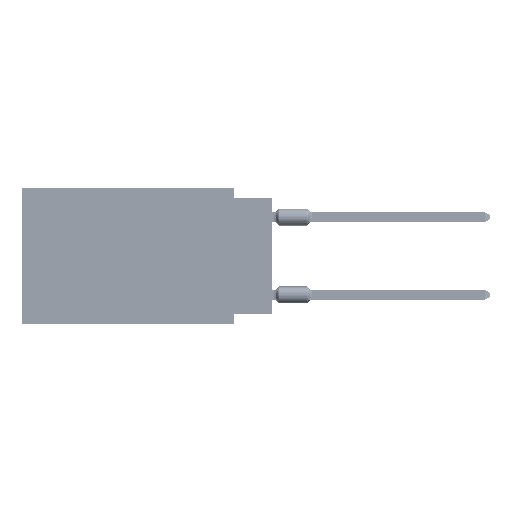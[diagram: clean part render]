
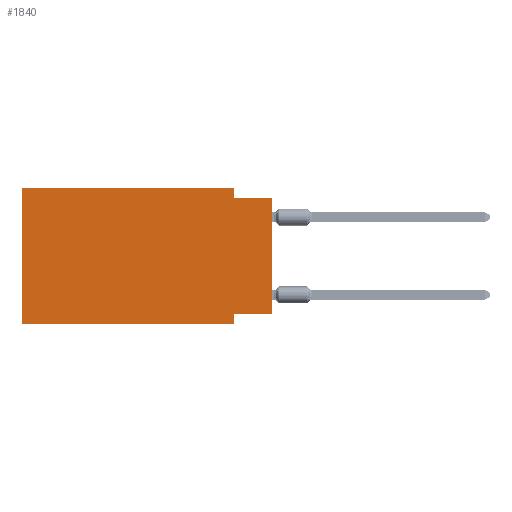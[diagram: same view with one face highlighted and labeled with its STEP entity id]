
A CAD part, left-side view. The second image highlights one B-rep face of the part: STEP entity #1840.
In plain terms, the highlighted planar face has unit normal (-1, 0, 0).
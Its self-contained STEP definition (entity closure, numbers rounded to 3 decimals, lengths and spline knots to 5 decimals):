
#1728 = DIRECTION ( 'NONE',  ( 0., 0., -1. ) ) ;
#1840 = ADVANCED_FACE ( 'NONE', ( #55163 ), #37522, .F. ) ;
#11171 = ORIENTED_EDGE ( 'NONE', *, *, #102995, .T. ) ;
#14180 = ORIENTED_EDGE ( 'NONE', *, *, #97804, .F. ) ;
#14461 = EDGE_CURVE ( 'NONE', #41664, #30178, #109440, .T. ) ;
#16264 = VERTEX_POINT ( 'NONE', #84594 ) ;
#18031 = DIRECTION ( 'NONE',  ( 0., 0., -1. ) ) ;
#18464 = CARTESIAN_POINT ( 'NONE',  ( 0., 0.645, -0.35 ) ) ;
#18963 = ORIENTED_EDGE ( 'NONE', *, *, #114320, .F. ) ;
#20844 = DIRECTION ( 'NONE',  ( 0., -1., 0. ) ) ;
#24533 = DIRECTION ( 'NONE',  ( 0., 1., 0. ) ) ;
#24712 = ORIENTED_EDGE ( 'NONE', *, *, #100279, .F. ) ;
#25217 = DIRECTION ( 'NONE',  ( 0., -1., 0. ) ) ;
#25830 = LINE ( 'NONE', #100045, #57787 ) ;
#27219 = VECTOR ( 'NONE', #100322, 39.37008 ) ;
#29696 = CARTESIAN_POINT ( 'NONE',  ( 0., 0.1, 0. ) ) ;
#30178 = VERTEX_POINT ( 'NONE', #80747 ) ;
#33663 = CARTESIAN_POINT ( 'NONE',  ( 0., 0.1, 0. ) ) ;
#34074 = AXIS2_PLACEMENT_3D ( 'NONE', #36300, #73372, #18031 ) ;
#36300 = CARTESIAN_POINT ( 'NONE',  ( 0., 0.645, 0. ) ) ;
#37522 = PLANE ( 'NONE',  #34074 ) ;
#37629 = CARTESIAN_POINT ( 'NONE',  ( 0., 0.1, -0.325 ) ) ;
#39136 = LINE ( 'NONE', #76215, #42806 ) ;
#41664 = VERTEX_POINT ( 'NONE', #37629 ) ;
#42806 = VECTOR ( 'NONE', #20844, 39.37008 ) ;
#43194 = LINE ( 'NONE', #118581, #103417 ) ;
#46558 = ORIENTED_EDGE ( 'NONE', *, *, #93673, .F. ) ;
#51172 = VECTOR ( 'NONE', #63378, 39.37008 ) ;
#54541 = ORIENTED_EDGE ( 'NONE', *, *, #88854, .F. ) ;
#55163 = FACE_OUTER_BOUND ( 'NONE', #103654, .T. ) ;
#56369 = DIRECTION ( 'NONE',  ( 0., 0., 1. ) ) ;
#56979 = LINE ( 'NONE', #57557, #110951 ) ;
#57087 = LINE ( 'NONE', #29696, #120132 ) ;
#57557 = CARTESIAN_POINT ( 'NONE',  ( 0., 0.645, 0. ) ) ;
#57787 = VECTOR ( 'NONE', #25217, 39.37008 ) ;
#59917 = VECTOR ( 'NONE', #24533, 39.37008 ) ;
#63378 = DIRECTION ( 'NONE',  ( 0., -1., 0. ) ) ;
#71627 = VERTEX_POINT ( 'NONE', #115306 ) ;
#71653 = VERTEX_POINT ( 'NONE', #80456 ) ;
#73372 = DIRECTION ( 'NONE',  ( 1., 0., 0. ) ) ;
#73404 = VERTEX_POINT ( 'NONE', #33663 ) ;
#73530 = CARTESIAN_POINT ( 'NONE',  ( 0., 0.1, -0.35 ) ) ;
#76215 = CARTESIAN_POINT ( 'NONE',  ( 0., 0.645, -0.35 ) ) ;
#79401 = VERTEX_POINT ( 'NONE', #18464 ) ;
#80456 = CARTESIAN_POINT ( 'NONE',  ( 0., 0., -0.025 ) ) ;
#80747 = CARTESIAN_POINT ( 'NONE',  ( 0., 0.1, -0.35 ) ) ;
#84594 = CARTESIAN_POINT ( 'NONE',  ( 0., 0.1, -0.025 ) ) ;
#85805 = ORIENTED_EDGE ( 'NONE', *, *, #14461, .F. ) ;
#88854 = EDGE_CURVE ( 'NONE', #79401, #101873, #56979, .T. ) ;
#88992 = CARTESIAN_POINT ( 'NONE',  ( 0., 0., -0.325 ) ) ;
#90009 = EDGE_CURVE ( 'NONE', #71627, #71653, #43194, .T. ) ;
#90148 = LINE ( 'NONE', #110820, #51172 ) ;
#91181 = ORIENTED_EDGE ( 'NONE', *, *, #90009, .T. ) ;
#93673 = EDGE_CURVE ( 'NONE', #16264, #71653, #90148, .T. ) ;
#97804 = EDGE_CURVE ( 'NONE', #101873, #73404, #25830, .T. ) ;
#100045 = CARTESIAN_POINT ( 'NONE',  ( 0., 0.645, 0. ) ) ;
#100279 = EDGE_CURVE ( 'NONE', #71627, #41664, #115772, .T. ) ;
#100322 = DIRECTION ( 'NONE',  ( 0., 0., -1. ) ) ;
#101873 = VERTEX_POINT ( 'NONE', #108316 ) ;
#102995 = EDGE_CURVE ( 'NONE', #79401, #30178, #39136, .T. ) ;
#103417 = VECTOR ( 'NONE', #117969, 39.37008 ) ;
#103654 = EDGE_LOOP ( 'NONE', ( #91181, #46558, #18963, #14180, #54541, #11171, #85805, #24712 ) ) ;
#108316 = CARTESIAN_POINT ( 'NONE',  ( 0., 0.645, 0. ) ) ;
#109440 = LINE ( 'NONE', #73530, #27219 ) ;
#110820 = CARTESIAN_POINT ( 'NONE',  ( 0., 0., -0.025 ) ) ;
#110951 = VECTOR ( 'NONE', #56369, 39.37008 ) ;
#114320 = EDGE_CURVE ( 'NONE', #73404, #16264, #57087, .T. ) ;
#115306 = CARTESIAN_POINT ( 'NONE',  ( 0., 0., -0.325 ) ) ;
#115772 = LINE ( 'NONE', #88992, #59917 ) ;
#117969 = DIRECTION ( 'NONE',  ( 0., 0., 1. ) ) ;
#118581 = CARTESIAN_POINT ( 'NONE',  ( 0., 0., 0. ) ) ;
#120132 = VECTOR ( 'NONE', #1728, 39.37008 ) ;
